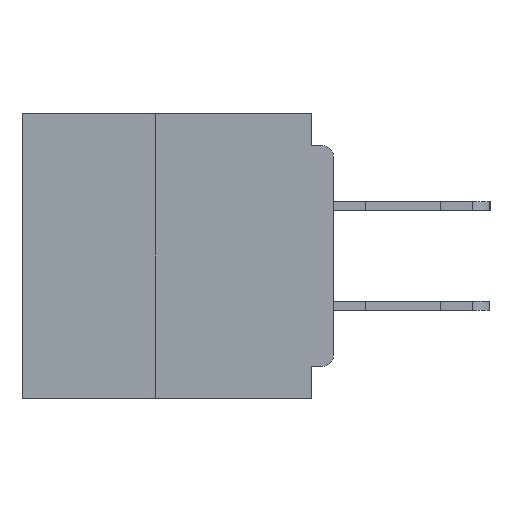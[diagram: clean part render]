
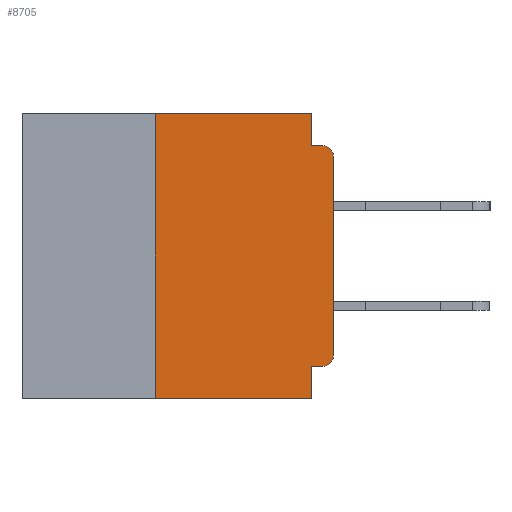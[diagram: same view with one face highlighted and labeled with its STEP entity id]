
A CAD part, left-side view. The second image highlights one B-rep face of the part: STEP entity #8705.
In plain terms, the highlighted planar face has unit normal (-1, 0, 0).
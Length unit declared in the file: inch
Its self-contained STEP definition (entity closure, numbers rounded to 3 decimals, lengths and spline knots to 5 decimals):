
#934 = VERTEX_POINT ( 'NONE', #25168 ) ;
#1117 = CIRCLE ( 'NONE', #27293, 0.015 ) ;
#1856 = EDGE_CURVE ( 'NONE', #33195, #22955, #51260, .T. ) ;
#2166 = VECTOR ( 'NONE', #28244, 39.37008 ) ;
#3377 = VERTEX_POINT ( 'NONE', #3940 ) ;
#3390 = VERTEX_POINT ( 'NONE', #4096 ) ;
#3940 = CARTESIAN_POINT ( 'NONE',  ( 0., 0.031, -0.045 ) ) ;
#4096 = CARTESIAN_POINT ( 'NONE',  ( 0., 0., -0.34 ) ) ;
#4150 = CARTESIAN_POINT ( 'NONE',  ( 0., 0., -0.045 ) ) ;
#4331 = VECTOR ( 'NONE', #14439, 39.37008 ) ;
#4473 = VECTOR ( 'NONE', #13088, 39.37008 ) ;
#4568 = EDGE_CURVE ( 'NONE', #39258, #22955, #49215, .T. ) ;
#4722 = VECTOR ( 'NONE', #47939, 39.37008 ) ;
#4939 = CARTESIAN_POINT ( 'NONE',  ( 0., 0., -0.355 ) ) ;
#4979 = EDGE_CURVE ( 'NONE', #3377, #934, #14133, .T. ) ;
#6339 = CARTESIAN_POINT ( 'NONE',  ( 0., 0.031, 0. ) ) ;
#7859 = VECTOR ( 'NONE', #48832, 39.37008 ) ;
#8705 = ADVANCED_FACE ( 'NONE', ( #43776 ), #29901, .F. ) ;
#9206 = CARTESIAN_POINT ( 'NONE',  ( 0., 0.015, -0.34 ) ) ;
#11347 = EDGE_CURVE ( 'NONE', #46470, #3390, #1117, .T. ) ;
#11913 = CARTESIAN_POINT ( 'NONE',  ( 0., 0.437, 0. ) ) ;
#12075 = LINE ( 'NONE', #14857, #45275 ) ;
#13031 = EDGE_CURVE ( 'NONE', #14416, #49835, #16692, .T. ) ;
#13088 = DIRECTION ( 'NONE',  ( 0., 0., 1. ) ) ;
#13110 = ORIENTED_EDGE ( 'NONE', *, *, #4568, .T. ) ;
#13273 = DIRECTION ( 'NONE',  ( 0., 0., -1. ) ) ;
#14038 = VECTOR ( 'NONE', #29005, 39.37008 ) ;
#14065 = ORIENTED_EDGE ( 'NONE', *, *, #4979, .F. ) ;
#14133 = LINE ( 'NONE', #4150, #2166 ) ;
#14416 = VERTEX_POINT ( 'NONE', #41232 ) ;
#14439 = DIRECTION ( 'NONE',  ( 0., 0., -1. ) ) ;
#14503 = VERTEX_POINT ( 'NONE', #38088 ) ;
#14857 = CARTESIAN_POINT ( 'NONE',  ( 0., 0.25, -0.4 ) ) ;
#15017 = LINE ( 'NONE', #6339, #4331 ) ;
#15344 = EDGE_CURVE ( 'NONE', #39258, #14416, #12075, .T. ) ;
#16692 = LINE ( 'NONE', #11913, #4722 ) ;
#16880 = CARTESIAN_POINT ( 'NONE',  ( 0., 0.437, -0.4 ) ) ;
#17659 = ORIENTED_EDGE ( 'NONE', *, *, #24791, .T. ) ;
#17978 = DIRECTION ( 'NONE',  ( 1., 0., 0. ) ) ;
#18056 = EDGE_CURVE ( 'NONE', #49835, #3377, #15017, .T. ) ;
#18863 = VECTOR ( 'NONE', #50559, 39.37008 ) ;
#20178 = AXIS2_PLACEMENT_3D ( 'NONE', #41920, #17978, #45911 ) ;
#21055 = ORIENTED_EDGE ( 'NONE', *, *, #1856, .F. ) ;
#21600 = CARTESIAN_POINT ( 'NONE',  ( 0., 0.031, 0. ) ) ;
#22955 = VERTEX_POINT ( 'NONE', #38149 ) ;
#23346 = ORIENTED_EDGE ( 'NONE', *, *, #37231, .T. ) ;
#23626 = DIRECTION ( 'NONE',  ( -1., 0., 0. ) ) ;
#24720 = LINE ( 'NONE', #4939, #14038 ) ;
#24791 = EDGE_CURVE ( 'NONE', #14503, #934, #45509, .T. ) ;
#25168 = CARTESIAN_POINT ( 'NONE',  ( 0., 0.015, -0.045 ) ) ;
#27293 = AXIS2_PLACEMENT_3D ( 'NONE', #9206, #37292, #13273 ) ;
#28244 = DIRECTION ( 'NONE',  ( 0., -1., 0. ) ) ;
#29005 = DIRECTION ( 'NONE',  ( 0., 1., 0. ) ) ;
#29901 = PLANE ( 'NONE',  #20178 ) ;
#30195 = EDGE_CURVE ( 'NONE', #46470, #33195, #24720, .T. ) ;
#33090 = CARTESIAN_POINT ( 'NONE',  ( 0., 0., 0. ) ) ;
#33114 = AXIS2_PLACEMENT_3D ( 'NONE', #47570, #23626, #51569 ) ;
#33195 = VERTEX_POINT ( 'NONE', #43508 ) ;
#35121 = ORIENTED_EDGE ( 'NONE', *, *, #13031, .F. ) ;
#37231 = EDGE_CURVE ( 'NONE', #3390, #14503, #47067, .T. ) ;
#37292 = DIRECTION ( 'NONE',  ( -1., 0., 0. ) ) ;
#38088 = CARTESIAN_POINT ( 'NONE',  ( 0., 0., -0.06 ) ) ;
#38149 = CARTESIAN_POINT ( 'NONE',  ( 0., 0.031, -0.4 ) ) ;
#39258 = VERTEX_POINT ( 'NONE', #39800 ) ;
#39800 = CARTESIAN_POINT ( 'NONE',  ( 0., 0.25, -0.4 ) ) ;
#40011 = ORIENTED_EDGE ( 'NONE', *, *, #30195, .F. ) ;
#41232 = CARTESIAN_POINT ( 'NONE',  ( 0., 0.25, 0. ) ) ;
#41920 = CARTESIAN_POINT ( 'NONE',  ( 0., 0.437, 0. ) ) ;
#42866 = DIRECTION ( 'NONE',  ( 0., 0., 1. ) ) ;
#43508 = CARTESIAN_POINT ( 'NONE',  ( 0., 0.031, -0.355 ) ) ;
#43776 = FACE_OUTER_BOUND ( 'NONE', #48003, .T. ) ;
#45275 = VECTOR ( 'NONE', #42866, 39.37008 ) ;
#45509 = CIRCLE ( 'NONE', #33114, 0.015 ) ;
#45911 = DIRECTION ( 'NONE',  ( 0., 0., -1. ) ) ;
#46218 = ORIENTED_EDGE ( 'NONE', *, *, #15344, .F. ) ;
#46470 = VERTEX_POINT ( 'NONE', #47516 ) ;
#46882 = ORIENTED_EDGE ( 'NONE', *, *, #11347, .T. ) ;
#47067 = LINE ( 'NONE', #33090, #4473 ) ;
#47516 = CARTESIAN_POINT ( 'NONE',  ( 0., 0.015, -0.355 ) ) ;
#47570 = CARTESIAN_POINT ( 'NONE',  ( 0., 0.015, -0.06 ) ) ;
#47939 = DIRECTION ( 'NONE',  ( 0., -1., 0. ) ) ;
#48003 = EDGE_LOOP ( 'NONE', ( #23346, #17659, #14065, #49223, #35121, #46218, #13110, #21055, #40011, #46882 ) ) ;
#48832 = DIRECTION ( 'NONE',  ( 0., -1., 0. ) ) ;
#49215 = LINE ( 'NONE', #16880, #7859 ) ;
#49223 = ORIENTED_EDGE ( 'NONE', *, *, #18056, .F. ) ;
#49835 = VERTEX_POINT ( 'NONE', #21600 ) ;
#50559 = DIRECTION ( 'NONE',  ( 0., 0., -1. ) ) ;
#50744 = CARTESIAN_POINT ( 'NONE',  ( 0., 0.031, -0.4 ) ) ;
#51260 = LINE ( 'NONE', #50744, #18863 ) ;
#51569 = DIRECTION ( 'NONE',  ( 0., 0., -1. ) ) ;
